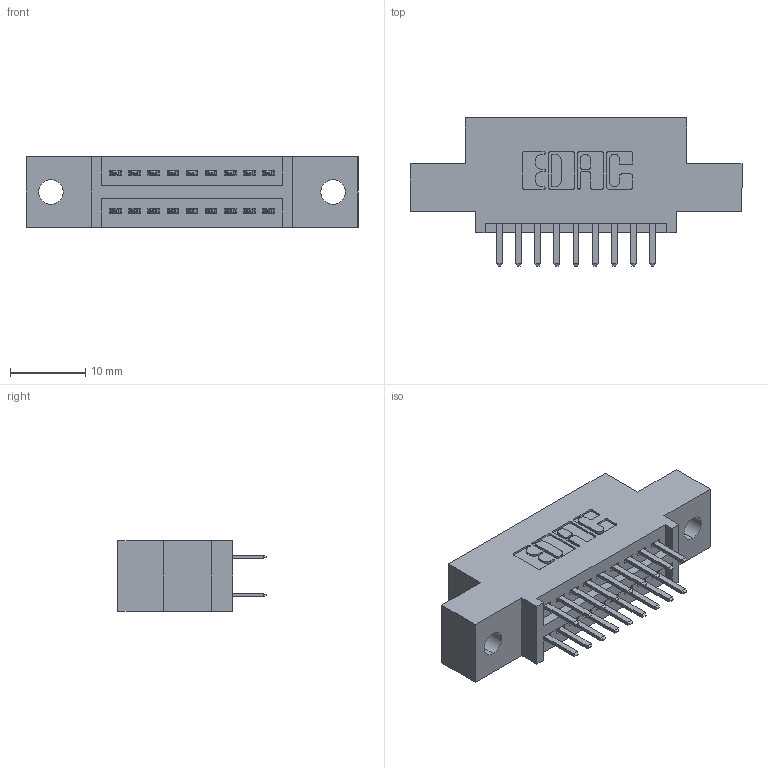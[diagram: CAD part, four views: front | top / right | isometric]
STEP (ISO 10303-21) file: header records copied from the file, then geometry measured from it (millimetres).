
FILE_DESCRIPTION (( 'STEP AP203' ), '1' );
FILE_NAME ('395-018-520-502.STEP', '2019-10-15T19:09:03', ( '' ), ( '' ), 'SwSTEP 2.0', 'SolidWorks 2016', '' );
FILE_SCHEMA (( 'CONFIG_CONTROL_DESIGN' ));
Length unit declared in the file: inch
Products named in the file (3): 345 Part_0.110 Offset - 0.128 Dia; 345-292-001_345-293-120; 395-018-520-502
Assembly tree (19 placements, depth 2):
  395-018-520-502
    345 Part_0.110 Offset - 0.128 Dia
    345-292-001_345-293-120  x18
Bounding box: 44.07 x 19.68 x 9.4 mm (x, y, z)
Volume: 3856.6 mm3; surface area: 4864.9 mm2
Topology: 19 solids, 19 shells, 1102 faces, 3179 edges, 2070 vertices
Faces by surface type: plane 714, cylinder 388
Entity records: 11753 total; most frequent: CARTESIAN_POINT 2016, ORIENTED_EDGE 1938, DIRECTION 1805, EDGE_CURVE 969, LINE 797, VECTOR 797, VERTEX_POINT 642, AXIS2_PLACEMENT_3D 504
